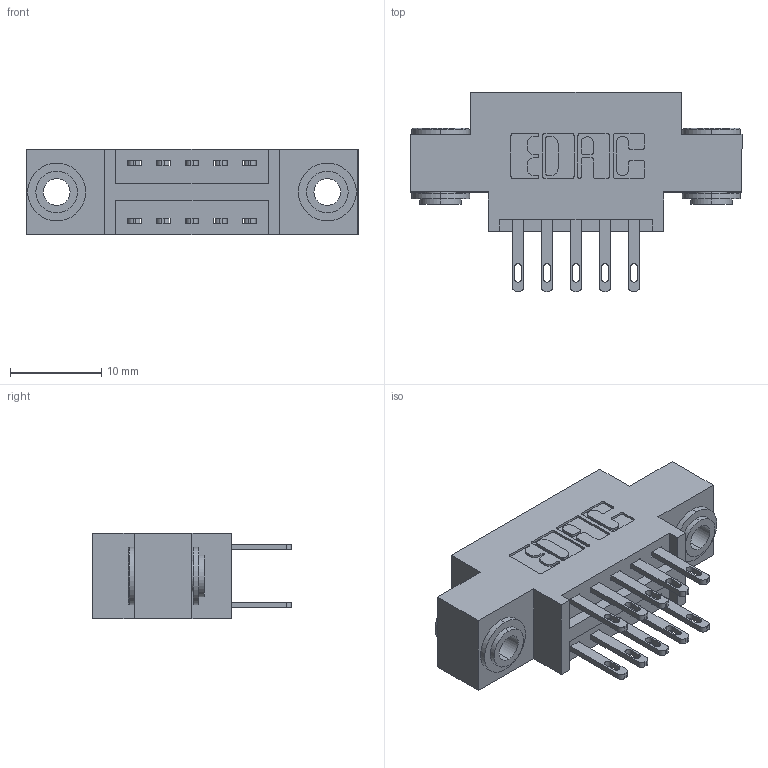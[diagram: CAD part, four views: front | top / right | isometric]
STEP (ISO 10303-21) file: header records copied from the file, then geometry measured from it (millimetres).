
FILE_DESCRIPTION (( 'STEP AP203' ), '1' );
FILE_NAME ('896-010-500-803.STEP', '2021-07-27T14:27:52', ( '' ), ( '' ), 'SwSTEP 2.0', 'SolidWorks 2020', '' );
FILE_SCHEMA (( 'CONFIG_CONTROL_DESIGN' ));
Length unit declared in the file: inch
Products named in the file (4): 345-292-001_345-293-100; 896-010-500-803; 846 Part_0.170 Offset - 0.156 Dia-TH; 345-250-002_345-250-002-102
Assembly tree (13 placements, depth 2):
  896-010-500-803
    846 Part_0.170 Offset - 0.156 Dia-TH
    345-292-001_345-293-100  x10
    345-250-002_345-250-002-102  x2
Bounding box: 36.45 x 21.84 x 9.4 mm (x, y, z)
Volume: 3162.2 mm3; surface area: 4263.6 mm2
Topology: 13 solids, 13 shells, 644 faces, 1887 edges, 1254 vertices
Faces by surface type: plane 380, cylinder 256, cone 8
Entity records: 8956 total; most frequent: CARTESIAN_POINT 1503, ORIENTED_EDGE 1430, DIRECTION 1409, EDGE_CURVE 715, VECTOR 535, LINE 535, VERTEX_POINT 474, AXIS2_PLACEMENT_3D 437
